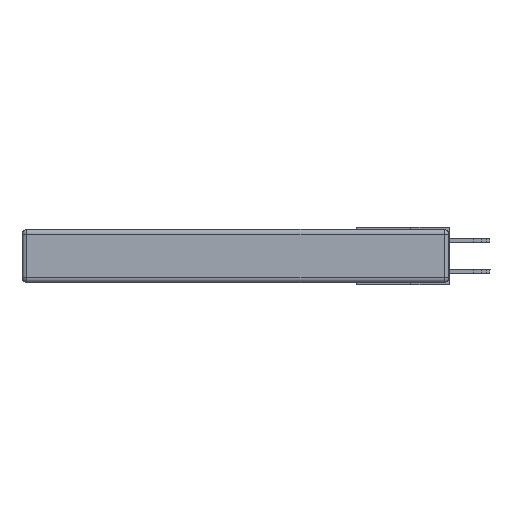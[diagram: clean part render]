
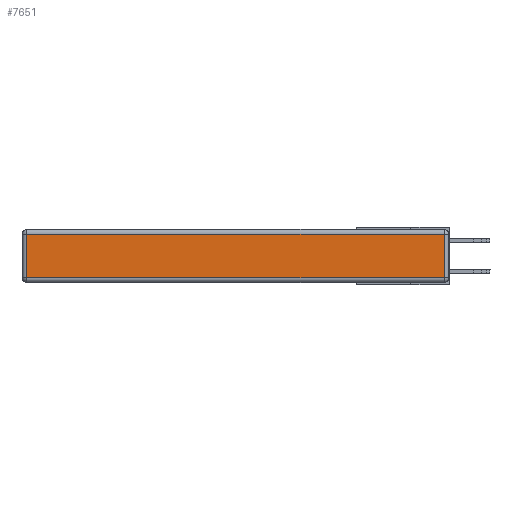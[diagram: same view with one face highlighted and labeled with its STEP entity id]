
A CAD part, left-side view. The second image highlights one B-rep face of the part: STEP entity #7651.
In plain terms, the highlighted planar face has unit normal (-1, 0, 0).
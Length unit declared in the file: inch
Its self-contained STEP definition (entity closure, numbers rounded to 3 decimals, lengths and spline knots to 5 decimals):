
#1092 = CARTESIAN_POINT ( 'NONE',  ( 0., 2.72, -0.03 ) ) ;
#1338 = VECTOR ( 'NONE', #20955, 39.37008 ) ;
#1831 = LINE ( 'NONE', #14989, #9900 ) ;
#2018 = VERTEX_POINT ( 'NONE', #11708 ) ;
#2248 = PLANE ( 'NONE',  #8870 ) ;
#2761 = DIRECTION ( 'NONE',  ( 0., -1., 0. ) ) ;
#3190 = ORIENTED_EDGE ( 'NONE', *, *, #4845, .T. ) ;
#4356 = VERTEX_POINT ( 'NONE', #1092 ) ;
#4845 = EDGE_CURVE ( 'NONE', #18080, #5841, #1831, .T. ) ;
#4944 = VECTOR ( 'NONE', #13466, 39.37008 ) ;
#5841 = VERTEX_POINT ( 'NONE', #16886 ) ;
#7651 = ADVANCED_FACE ( 'NONE', ( #20989 ), #2248, .T. ) ;
#7962 = ORIENTED_EDGE ( 'NONE', *, *, #12202, .T. ) ;
#8772 = EDGE_LOOP ( 'NONE', ( #10372, #3190, #18585, #7962 ) ) ;
#8870 = AXIS2_PLACEMENT_3D ( 'NONE', #12333, #17223, #18740 ) ;
#9537 = LINE ( 'NONE', #12431, #17708 ) ;
#9606 = EDGE_CURVE ( 'NONE', #2018, #18080, #9537, .T. ) ;
#9900 = VECTOR ( 'NONE', #17985, 39.37008 ) ;
#10372 = ORIENTED_EDGE ( 'NONE', *, *, #9606, .T. ) ;
#11708 = CARTESIAN_POINT ( 'NONE',  ( 0., 2.72, -0.313 ) ) ;
#12008 = CARTESIAN_POINT ( 'NONE',  ( 0., 2.75, -0.03 ) ) ;
#12202 = EDGE_CURVE ( 'NONE', #4356, #2018, #17591, .T. ) ;
#12333 = CARTESIAN_POINT ( 'NONE',  ( 0., 0., -0.343 ) ) ;
#12431 = CARTESIAN_POINT ( 'NONE',  ( 0., 0., -0.313 ) ) ;
#13466 = DIRECTION ( 'NONE',  ( 0., 1., 0. ) ) ;
#14604 = CARTESIAN_POINT ( 'NONE',  ( 0., 2.72, -0.343 ) ) ;
#14989 = CARTESIAN_POINT ( 'NONE',  ( 0., 0.03, -0.343 ) ) ;
#15854 = LINE ( 'NONE', #12008, #4944 ) ;
#16018 = EDGE_CURVE ( 'NONE', #5841, #4356, #15854, .T. ) ;
#16118 = CARTESIAN_POINT ( 'NONE',  ( 0., 0.03, -0.313 ) ) ;
#16886 = CARTESIAN_POINT ( 'NONE',  ( 0., 0.03, -0.03 ) ) ;
#17223 = DIRECTION ( 'NONE',  ( -1., 0., 0. ) ) ;
#17591 = LINE ( 'NONE', #14604, #1338 ) ;
#17708 = VECTOR ( 'NONE', #2761, 39.37008 ) ;
#17985 = DIRECTION ( 'NONE',  ( 0., 0., 1. ) ) ;
#18080 = VERTEX_POINT ( 'NONE', #16118 ) ;
#18585 = ORIENTED_EDGE ( 'NONE', *, *, #16018, .T. ) ;
#18740 = DIRECTION ( 'NONE',  ( 0., 0., 1. ) ) ;
#20955 = DIRECTION ( 'NONE',  ( 0., 0., -1. ) ) ;
#20989 = FACE_OUTER_BOUND ( 'NONE', #8772, .T. ) ;
